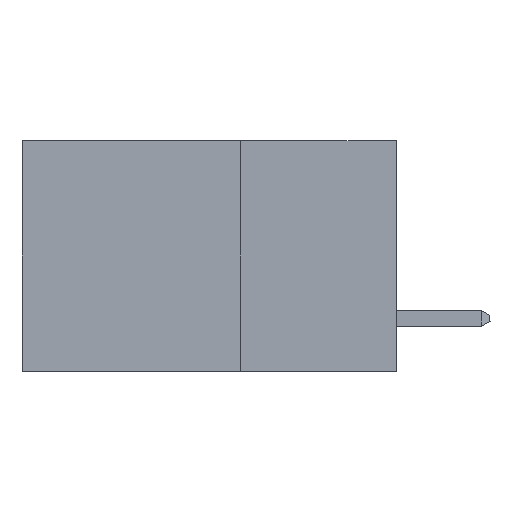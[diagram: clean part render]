
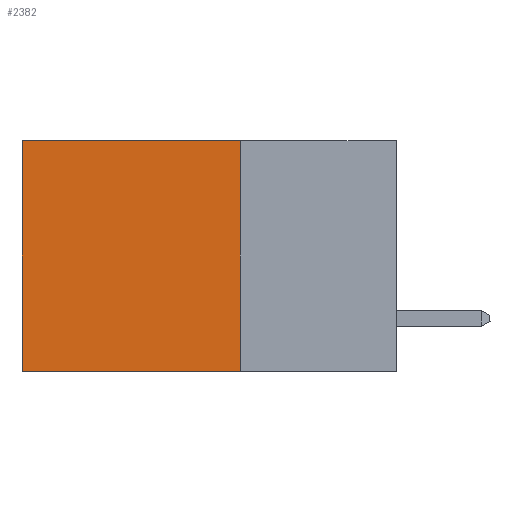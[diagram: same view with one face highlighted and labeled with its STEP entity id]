
A CAD part, left-side view. The second image highlights one B-rep face of the part: STEP entity #2382.
In plain terms, the highlighted planar face has unit normal (-1, 0, 0).
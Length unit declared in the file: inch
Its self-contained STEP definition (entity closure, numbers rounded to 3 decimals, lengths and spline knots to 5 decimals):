
#768 = VECTOR ( 'NONE', #6184, 39.37008 ) ;
#1306 = CARTESIAN_POINT ( 'NONE',  ( 0.298, 0.25, -0.37 ) ) ;
#2382 = ADVANCED_FACE ( 'NONE', ( #6844 ), #22013, .F. ) ;
#2676 = AXIS2_PLACEMENT_3D ( 'NONE', #19930, #21911, #12601 ) ;
#3098 = VERTEX_POINT ( 'NONE', #1306 ) ;
#4778 = LINE ( 'NONE', #15613, #768 ) ;
#5902 = EDGE_CURVE ( 'NONE', #24104, #25888, #6935, .T. ) ;
#6184 = DIRECTION ( 'NONE',  ( 0., 1., 0. ) ) ;
#6844 = FACE_OUTER_BOUND ( 'NONE', #9212, .T. ) ;
#6935 = LINE ( 'NONE', #22580, #12505 ) ;
#7557 = ORIENTED_EDGE ( 'NONE', *, *, #23200, .T. ) ;
#9212 = EDGE_LOOP ( 'NONE', ( #23035, #16376, #24623, #7557 ) ) ;
#9582 = CARTESIAN_POINT ( 'NONE',  ( 0.298, 0.25, 0. ) ) ;
#11246 = EDGE_CURVE ( 'NONE', #28031, #3098, #26646, .T. ) ;
#12505 = VECTOR ( 'NONE', #22483, 39.37008 ) ;
#12601 = DIRECTION ( 'NONE',  ( 0., 0., -1. ) ) ;
#15354 = CARTESIAN_POINT ( 'NONE',  ( 0.298, 0.6, -0.37 ) ) ;
#15613 = CARTESIAN_POINT ( 'NONE',  ( 0.298, 0.25, -0.37 ) ) ;
#16376 = ORIENTED_EDGE ( 'NONE', *, *, #17416, .F. ) ;
#17416 = EDGE_CURVE ( 'NONE', #3098, #25888, #4778, .T. ) ;
#19930 = CARTESIAN_POINT ( 'NONE',  ( 0.298, 0.25, 0. ) ) ;
#20377 = DIRECTION ( 'NONE',  ( 0., 1., 0. ) ) ;
#21911 = DIRECTION ( 'NONE',  ( 1., 0., 0. ) ) ;
#22013 = PLANE ( 'NONE',  #2676 ) ;
#22406 = VECTOR ( 'NONE', #20377, 39.37008 ) ;
#22483 = DIRECTION ( 'NONE',  ( 0., 0., -1. ) ) ;
#22580 = CARTESIAN_POINT ( 'NONE',  ( 0.298, 0.6, 0. ) ) ;
#22964 = VECTOR ( 'NONE', #25997, 39.37008 ) ;
#23035 = ORIENTED_EDGE ( 'NONE', *, *, #5902, .T. ) ;
#23200 = EDGE_CURVE ( 'NONE', #28031, #24104, #28314, .T. ) ;
#24104 = VERTEX_POINT ( 'NONE', #26124 ) ;
#24623 = ORIENTED_EDGE ( 'NONE', *, *, #11246, .F. ) ;
#25888 = VERTEX_POINT ( 'NONE', #15354 ) ;
#25997 = DIRECTION ( 'NONE',  ( 0., 0., -1. ) ) ;
#26124 = CARTESIAN_POINT ( 'NONE',  ( 0.298, 0.6, 0. ) ) ;
#26646 = LINE ( 'NONE', #28371, #22964 ) ;
#28031 = VERTEX_POINT ( 'NONE', #9582 ) ;
#28314 = LINE ( 'NONE', #29673, #22406 ) ;
#28371 = CARTESIAN_POINT ( 'NONE',  ( 0.298, 0.25, 0. ) ) ;
#29673 = CARTESIAN_POINT ( 'NONE',  ( 0.298, 0.25, 0. ) ) ;
